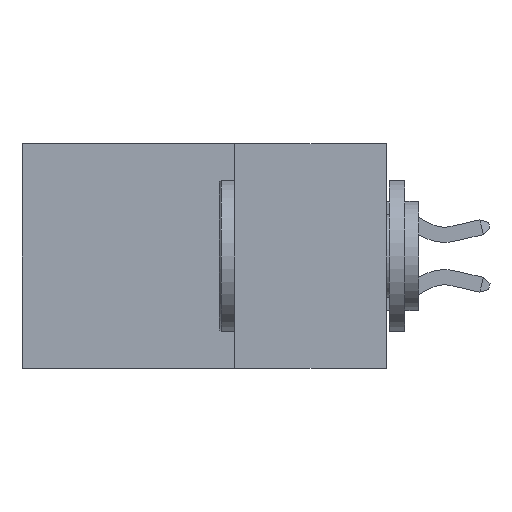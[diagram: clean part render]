
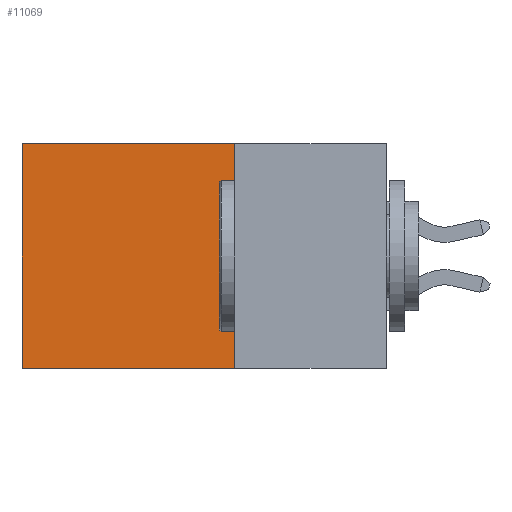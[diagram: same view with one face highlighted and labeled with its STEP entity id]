
A CAD part, left-side view. The second image highlights one B-rep face of the part: STEP entity #11069.
In plain terms, the highlighted planar face has unit normal (-1, 0, 0).
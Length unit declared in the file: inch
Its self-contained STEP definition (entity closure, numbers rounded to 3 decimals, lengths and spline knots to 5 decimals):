
#296 = VECTOR ( 'NONE', #9948, 39.37008 ) ;
#573 = EDGE_CURVE ( 'NONE', #7346, #4491, #9435, .T. ) ;
#609 = LINE ( 'NONE', #12059, #296 ) ;
#860 = ORIENTED_EDGE ( 'NONE', *, *, #7069, .T. ) ;
#921 = CARTESIAN_POINT ( 'NONE',  ( 0.2615, 0.25, -0.37 ) ) ;
#1230 = DIRECTION ( 'NONE',  ( 0., 0., -1. ) ) ;
#1246 = CARTESIAN_POINT ( 'NONE',  ( 0.2615, 0.6, -0.37 ) ) ;
#1316 = DIRECTION ( 'NONE',  ( 0., 1., 0. ) ) ;
#1641 = EDGE_LOOP ( 'NONE', ( #11671, #9747, #8017, #860 ) ) ;
#1933 = DIRECTION ( 'NONE',  ( 1., 0., 0. ) ) ;
#2095 = VERTEX_POINT ( 'NONE', #3929 ) ;
#2508 = DIRECTION ( 'NONE',  ( 0., 0., -1. ) ) ;
#2597 = AXIS2_PLACEMENT_3D ( 'NONE', #7738, #1933, #8718 ) ;
#3757 = LINE ( 'NONE', #1246, #8257 ) ;
#3929 = CARTESIAN_POINT ( 'NONE',  ( 0.2615, 0.25, 0. ) ) ;
#4086 = CARTESIAN_POINT ( 'NONE',  ( 0.2615, 0.6, 0. ) ) ;
#4123 = VECTOR ( 'NONE', #2508, 39.37008 ) ;
#4450 = CARTESIAN_POINT ( 'NONE',  ( 0.2615, 0.25, -0.37 ) ) ;
#4491 = VERTEX_POINT ( 'NONE', #5674 ) ;
#5674 = CARTESIAN_POINT ( 'NONE',  ( 0.2615, 0.6, -0.37 ) ) ;
#6663 = LINE ( 'NONE', #4450, #4123 ) ;
#6837 = EDGE_CURVE ( 'NONE', #8733, #4491, #3757, .T. ) ;
#6936 = FACE_OUTER_BOUND ( 'NONE', #1641, .T. ) ;
#7069 = EDGE_CURVE ( 'NONE', #2095, #8733, #609, .T. ) ;
#7346 = VERTEX_POINT ( 'NONE', #8440 ) ;
#7738 = CARTESIAN_POINT ( 'NONE',  ( 0.2615, 0.25, -0.37 ) ) ;
#8017 = ORIENTED_EDGE ( 'NONE', *, *, #9522, .F. ) ;
#8257 = VECTOR ( 'NONE', #1230, 39.37008 ) ;
#8440 = CARTESIAN_POINT ( 'NONE',  ( 0.2615, 0.25, -0.37 ) ) ;
#8718 = DIRECTION ( 'NONE',  ( 0., 0., -1. ) ) ;
#8733 = VERTEX_POINT ( 'NONE', #4086 ) ;
#9435 = LINE ( 'NONE', #921, #11908 ) ;
#9522 = EDGE_CURVE ( 'NONE', #2095, #7346, #6663, .T. ) ;
#9747 = ORIENTED_EDGE ( 'NONE', *, *, #573, .F. ) ;
#9948 = DIRECTION ( 'NONE',  ( 0., 1., 0. ) ) ;
#11069 = ADVANCED_FACE ( 'NONE', ( #6936 ), #12432, .F. ) ;
#11671 = ORIENTED_EDGE ( 'NONE', *, *, #6837, .T. ) ;
#11908 = VECTOR ( 'NONE', #1316, 39.37008 ) ;
#12059 = CARTESIAN_POINT ( 'NONE',  ( 0.2615, 0.25, 0. ) ) ;
#12432 = PLANE ( 'NONE',  #2597 ) ;
